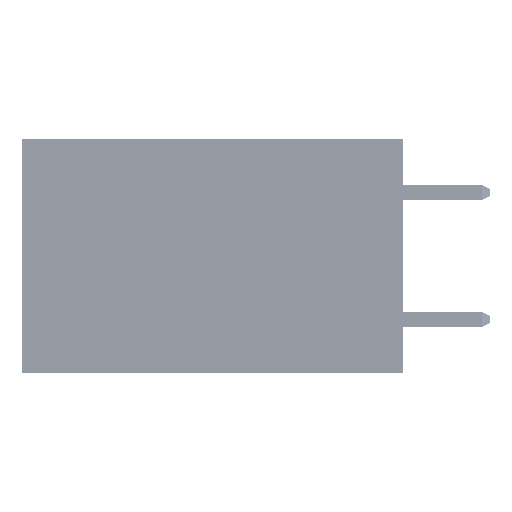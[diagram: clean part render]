
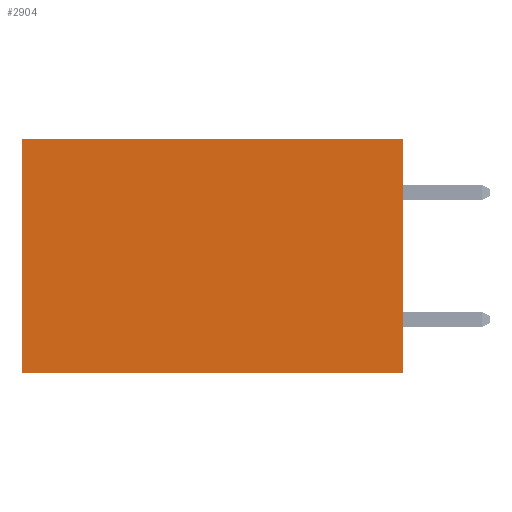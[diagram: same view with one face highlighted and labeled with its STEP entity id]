
A CAD part, left-side view. The second image highlights one B-rep face of the part: STEP entity #2904.
In plain terms, the highlighted planar face has unit normal (-1, 0, 0).
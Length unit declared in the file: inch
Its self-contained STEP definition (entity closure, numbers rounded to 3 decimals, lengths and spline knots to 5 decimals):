
#2245 = ORIENTED_EDGE ( 'NONE', *, *, #43471, .F. ) ;
#2904 = ADVANCED_FACE ( 'NONE', ( #22789 ), #30571, .F. ) ;
#3966 = DIRECTION ( 'NONE',  ( 0., 0., -1. ) ) ;
#7590 = ORIENTED_EDGE ( 'NONE', *, *, #45119, .T. ) ;
#8481 = DIRECTION ( 'NONE',  ( 0., 0., -1. ) ) ;
#8976 = AXIS2_PLACEMENT_3D ( 'NONE', #48529, #18803, #24748 ) ;
#9414 = LINE ( 'NONE', #34347, #30670 ) ;
#9814 = CARTESIAN_POINT ( 'NONE',  ( 0.2875, 0., -0.37 ) ) ;
#13089 = VECTOR ( 'NONE', #31934, 39.37008 ) ;
#13163 = CARTESIAN_POINT ( 'NONE',  ( 0.2875, 0., 0. ) ) ;
#15024 = EDGE_CURVE ( 'NONE', #28467, #45595, #44416, .T. ) ;
#16041 = EDGE_LOOP ( 'NONE', ( #7590, #30301, #2245, #34830 ) ) ;
#18341 = CARTESIAN_POINT ( 'NONE',  ( 0.2875, 0.6, 0. ) ) ;
#18394 = CARTESIAN_POINT ( 'NONE',  ( 0.2875, 0., -0.37 ) ) ;
#18803 = DIRECTION ( 'NONE',  ( 1., 0., 0. ) ) ;
#18990 = VECTOR ( 'NONE', #27254, 39.37008 ) ;
#19464 = EDGE_CURVE ( 'NONE', #22198, #34180, #23098, .T. ) ;
#19858 = CARTESIAN_POINT ( 'NONE',  ( 0.2875, 0., 0. ) ) ;
#21743 = CARTESIAN_POINT ( 'NONE',  ( 0.2875, 0.6, -0.37 ) ) ;
#22198 = VERTEX_POINT ( 'NONE', #13163 ) ;
#22789 = FACE_OUTER_BOUND ( 'NONE', #16041, .T. ) ;
#23098 = LINE ( 'NONE', #42460, #18990 ) ;
#24748 = DIRECTION ( 'NONE',  ( 0., 0., -1. ) ) ;
#26108 = VECTOR ( 'NONE', #8481, 39.37008 ) ;
#27254 = DIRECTION ( 'NONE',  ( 0., 1., 0. ) ) ;
#28467 = VERTEX_POINT ( 'NONE', #18394 ) ;
#30301 = ORIENTED_EDGE ( 'NONE', *, *, #15024, .F. ) ;
#30571 = PLANE ( 'NONE',  #8976 ) ;
#30670 = VECTOR ( 'NONE', #3966, 39.37008 ) ;
#31934 = DIRECTION ( 'NONE',  ( 0., 1., 0. ) ) ;
#34180 = VERTEX_POINT ( 'NONE', #18341 ) ;
#34347 = CARTESIAN_POINT ( 'NONE',  ( 0.2875, 0.6, 0. ) ) ;
#34830 = ORIENTED_EDGE ( 'NONE', *, *, #19464, .T. ) ;
#34987 = LINE ( 'NONE', #19858, #26108 ) ;
#42460 = CARTESIAN_POINT ( 'NONE',  ( 0.2875, 0., 0. ) ) ;
#43471 = EDGE_CURVE ( 'NONE', #22198, #28467, #34987, .T. ) ;
#44416 = LINE ( 'NONE', #9814, #13089 ) ;
#45119 = EDGE_CURVE ( 'NONE', #34180, #45595, #9414, .T. ) ;
#45595 = VERTEX_POINT ( 'NONE', #21743 ) ;
#48529 = CARTESIAN_POINT ( 'NONE',  ( 0.2875, 0., 0. ) ) ;
